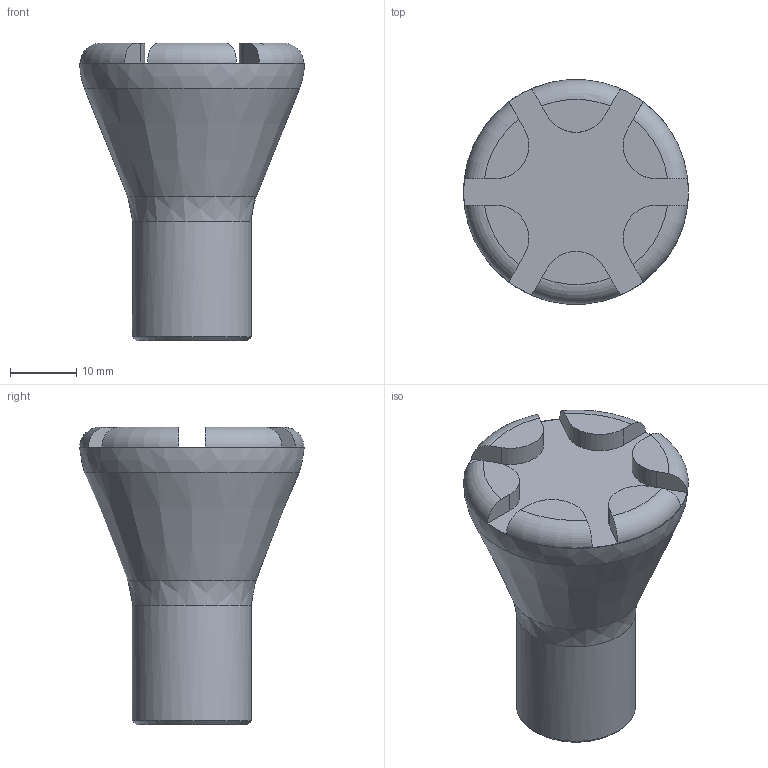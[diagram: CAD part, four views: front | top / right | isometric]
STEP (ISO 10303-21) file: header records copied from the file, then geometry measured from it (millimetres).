
FILE_DESCRIPTION(('FreeCAD Model'),'2;1');
FILE_NAME('Open CASCADE Shape Model','2022-10-05T16:46:39',('Author'),( ''),'Open CASCADE STEP processor 7.6','FreeCAD','Unknown');
FILE_SCHEMA(('AUTOMOTIVE_DESIGN { 1 0 10303 214 1 1 1 1 }'));
Length unit declared in the file: millimetre
Products named in the file (1): Pusher
Bounding box: 34 x 33.96 x 45 mm (x, y, z)
Volume: 19005.1 mm3; surface area: 4712.6 mm2
Topology: 1 solids, 1 shells, 38 faces, 91 edges, 55 vertices
Faces by surface type: plane 20, cylinder 8, torus 6, bspline 2, cone 2
Full cylindrical faces by diameter (mm): 18 x1, 34 x1
Entity records: 3039 total; most frequent: CARTESIAN_POINT 1245, DIRECTION 322, ORIENTED_EDGE 182, PCURVE 182, DEFINITIONAL_REPRESENTATION 182, LINE 162, VECTOR 162, EDGE_CURVE 91
